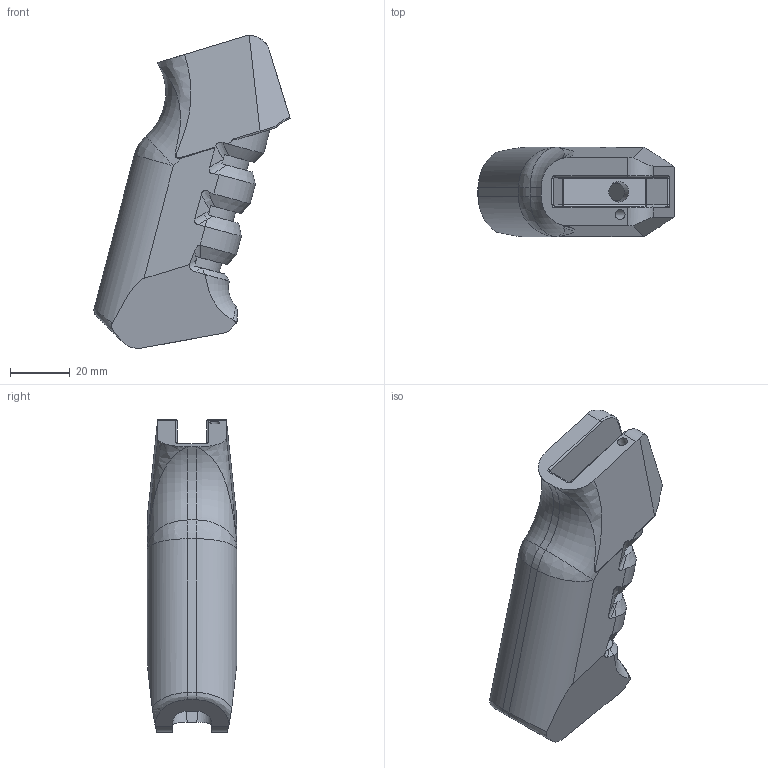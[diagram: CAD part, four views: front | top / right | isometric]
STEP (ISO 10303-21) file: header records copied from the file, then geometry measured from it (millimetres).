
FILE_DESCRIPTION(/* description */ (''),/* implementation_level */ '2;1');
FILE_NAME(/* name */ 'Pistol Grip .step',/* time_stamp */ '2022-05-12T10:56:02-06:00',/* author */ (''),/* organization */ (''),/* preprocessor_version */ 'ST-DEVELOPER v18.1',/* originating_system */ 'Autodesk Translation Framework v10.10.0.1391',/* authorisation */ '');
FILE_SCHEMA (('AUTOMOTIVE_DESIGN { 1 0 10303 214 3 1 1 }'));
Length unit declared in the file: millimetre
Products named in the file (1): Pistol Grip (1)
Bounding box: 65.38 x 29.84 x 104.3 mm (x, y, z)
Volume: 63493.5 mm3; surface area: 21791.7 mm2
Topology: 1 solids, 1 shells, 179 faces, 476 edges, 296 vertices
Faces by surface type: plane 63, cylinder 51, bspline 38, cone 13, torus 10, sphere 4
Full cylindrical faces by diameter (mm): 3.4 x1, 6.8 x1
Entity records: 7302 total; most frequent: CARTESIAN_POINT 3147, ORIENTED_EDGE 944, DIRECTION 747, EDGE_CURVE 472, VERTEX_POINT 296, AXIS2_PLACEMENT_3D 280, LINE 187, VECTOR 187
